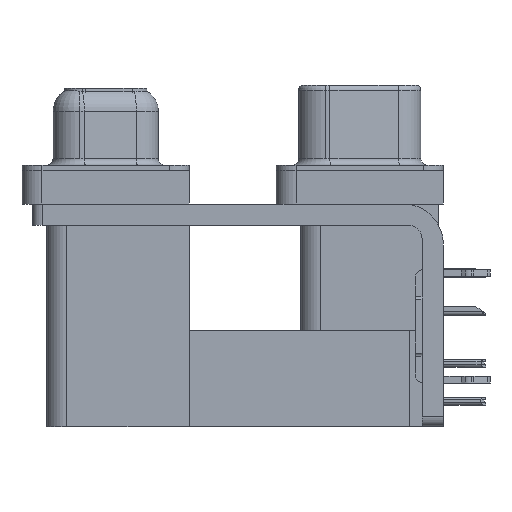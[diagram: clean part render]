
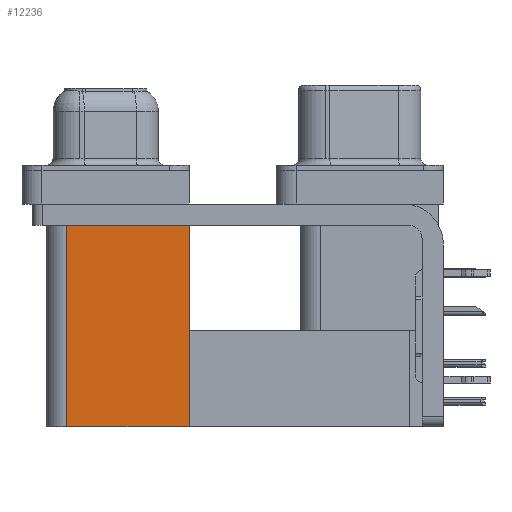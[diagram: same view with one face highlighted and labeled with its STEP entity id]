
A CAD part, left-side view. The second image highlights one B-rep face of the part: STEP entity #12236.
In plain terms, the highlighted planar face has unit normal (-1, 0, 0).
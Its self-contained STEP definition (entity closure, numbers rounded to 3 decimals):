
#394 = VECTOR ( 'NONE', #34885, 1000. ) ;
#2714 = EDGE_CURVE ( 'NONE', #35609, #19207, #31789, .T. ) ;
#2991 = CARTESIAN_POINT ( 'NONE',  ( 3.765, 21.975, -2.5 ) ) ;
#4614 = VERTEX_POINT ( 'NONE', #27313 ) ;
#5331 = EDGE_CURVE ( 'NONE', #36055, #35609, #43744, .T. ) ;
#5981 = EDGE_CURVE ( 'NONE', #36055, #4614, #16488, .T. ) ;
#6550 = CARTESIAN_POINT ( 'NONE',  ( 3.765, 21.975, -19.2 ) ) ;
#8935 = DIRECTION ( 'NONE',  ( 0., 0., 1. ) ) ;
#12236 = ADVANCED_FACE ( 'NONE', ( #26008 ), #23413, .F. ) ;
#13697 = CARTESIAN_POINT ( 'NONE',  ( 3.765, 12.775, -2.5 ) ) ;
#15640 = DIRECTION ( 'NONE',  ( 1., 0., 0. ) ) ;
#16488 = LINE ( 'NONE', #26835, #32367 ) ;
#19207 = VERTEX_POINT ( 'NONE', #2991 ) ;
#20111 = VECTOR ( 'NONE', #35885, 1000. ) ;
#22215 = CARTESIAN_POINT ( 'NONE',  ( 3.765, 12.775, -19.2 ) ) ;
#23413 = PLANE ( 'NONE',  #31738 ) ;
#26008 = FACE_OUTER_BOUND ( 'NONE', #32247, .T. ) ;
#26835 = CARTESIAN_POINT ( 'NONE',  ( 3.765, 12.775, -19.2 ) ) ;
#27313 = CARTESIAN_POINT ( 'NONE',  ( 3.765, 12.775, -2.5 ) ) ;
#30038 = DIRECTION ( 'NONE',  ( 0., 1., 0. ) ) ;
#30233 = DIRECTION ( 'NONE',  ( 0., 1., 0. ) ) ;
#30826 = EDGE_CURVE ( 'NONE', #4614, #19207, #46090, .T. ) ;
#31738 = AXIS2_PLACEMENT_3D ( 'NONE', #37364, #15640, #30038 ) ;
#31789 = LINE ( 'NONE', #6550, #394 ) ;
#32247 = EDGE_LOOP ( 'NONE', ( #46436, #43183, #43589, #38094 ) ) ;
#32367 = VECTOR ( 'NONE', #8935, 1000. ) ;
#34885 = DIRECTION ( 'NONE',  ( 0., 0., 1. ) ) ;
#35609 = VERTEX_POINT ( 'NONE', #45561 ) ;
#35885 = DIRECTION ( 'NONE',  ( 0., 1., 0. ) ) ;
#36055 = VERTEX_POINT ( 'NONE', #40427 ) ;
#37364 = CARTESIAN_POINT ( 'NONE',  ( 3.765, 12.775, -19.2 ) ) ;
#38094 = ORIENTED_EDGE ( 'NONE', *, *, #5981, .T. ) ;
#40427 = CARTESIAN_POINT ( 'NONE',  ( 3.765, 12.775, -19.2 ) ) ;
#43183 = ORIENTED_EDGE ( 'NONE', *, *, #2714, .F. ) ;
#43589 = ORIENTED_EDGE ( 'NONE', *, *, #5331, .F. ) ;
#43744 = LINE ( 'NONE', #22215, #46694 ) ;
#45561 = CARTESIAN_POINT ( 'NONE',  ( 3.765, 21.975, -19.2 ) ) ;
#46090 = LINE ( 'NONE', #13697, #20111 ) ;
#46436 = ORIENTED_EDGE ( 'NONE', *, *, #30826, .T. ) ;
#46694 = VECTOR ( 'NONE', #30233, 1000. ) ;
